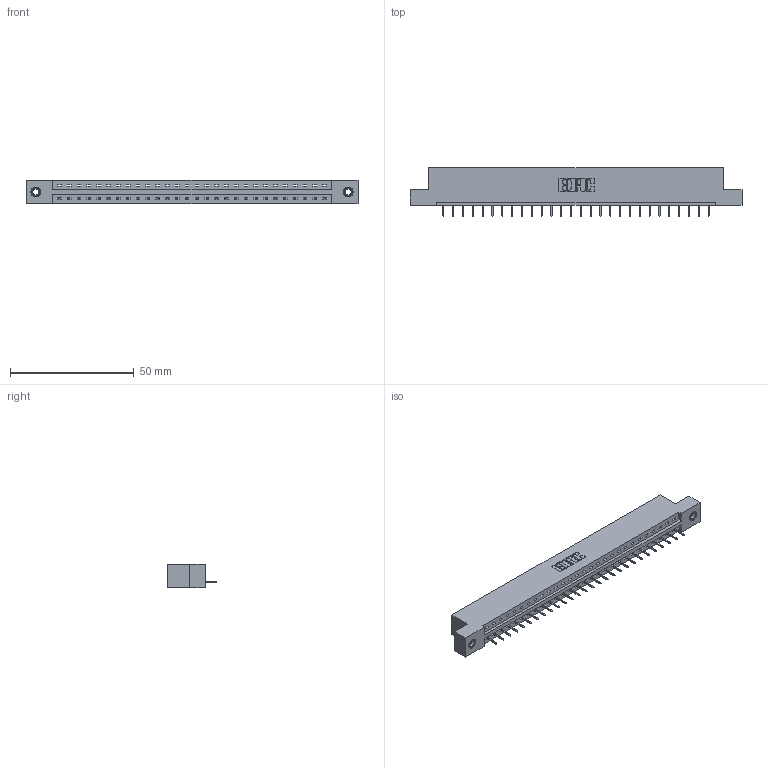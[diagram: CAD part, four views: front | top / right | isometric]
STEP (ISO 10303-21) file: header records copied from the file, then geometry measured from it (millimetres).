
FILE_DESCRIPTION (( 'STEP AP203' ), '1' );
FILE_NAME ('387-028-524-107.STEP', '2019-10-03T16:06:17', ( '' ), ( '' ), 'SwSTEP 2.0', 'SolidWorks 2016', '' );
FILE_SCHEMA (( 'CONFIG_CONTROL_DESIGN' ));
Length unit declared in the file: inch
Products named in the file (4): 345-250-001_345-250-005-103; 387-028-524-107; 337 Part_Flush Mounting Lugs - 0.156 Dia-TI; 345-292-001_345-293-124
Assembly tree (31 placements, depth 2):
  387-028-524-107
    337 Part_Flush Mounting Lugs - 0.156 Dia-TI
    345-292-001_345-293-124  x28
    345-250-001_345-250-005-103  x2
Bounding box: 133.96 x 19.69 x 9.4 mm (x, y, z)
Volume: 13623.5 mm3; surface area: 13652.3 mm2
Topology: 31 solids, 31 shells, 2022 faces, 5823 edges, 3762 vertices
Faces by surface type: plane 1558, cylinder 448, cone 12, torus 4
Entity records: 23884 total; most frequent: CARTESIAN_POINT 4137, ORIENTED_EDGE 4094, DIRECTION 3545, EDGE_CURVE 2047, VECTOR 1903, LINE 1903, VERTEX_POINT 1356, AXIS2_PLACEMENT_3D 821
